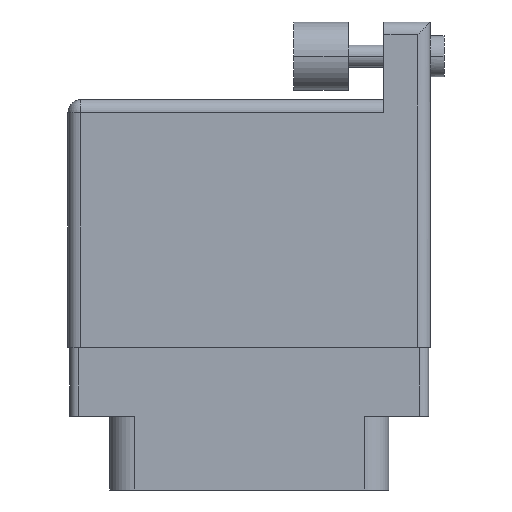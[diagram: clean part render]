
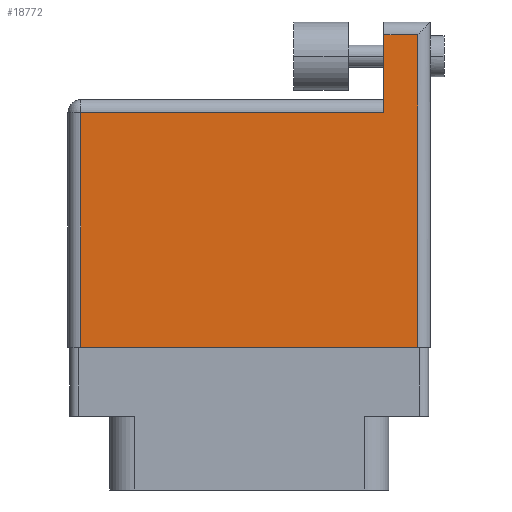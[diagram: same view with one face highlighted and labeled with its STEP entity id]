
A CAD part, front view. The second image highlights one B-rep face of the part: STEP entity #18772.
In plain terms, the highlighted face is planar.
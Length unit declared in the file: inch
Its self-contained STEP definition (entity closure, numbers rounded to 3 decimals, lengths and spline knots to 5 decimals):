
#295 = CARTESIAN_POINT ( 'NONE',  ( 0., 0.859, 0. ) ) ;
#579 = LINE ( 'NONE', #4725, #26224 ) ;
#1175 = CARTESIAN_POINT ( 'NONE',  ( 1.155, 0.859, 0. ) ) ;
#1245 = ORIENTED_EDGE ( 'NONE', *, *, #17087, .T. ) ;
#1353 = EDGE_LOOP ( 'NONE', ( #15851, #1245, #9022, #12493, #11175, #5600 ) ) ;
#1596 = LINE ( 'NONE', #13975, #12125 ) ;
#2258 = EDGE_CURVE ( 'NONE', #20447, #18096, #12729, .T. ) ;
#2852 = EDGE_CURVE ( 'NONE', #18024, #20447, #10308, .T. ) ;
#2933 = VECTOR ( 'NONE', #10618, 39.37008 ) ;
#4389 = EDGE_CURVE ( 'NONE', #18096, #18559, #22973, .T. ) ;
#4429 = DIRECTION ( 'NONE',  ( -1., 0., 0. ) ) ;
#4568 = VERTEX_POINT ( 'NONE', #19493 ) ;
#4725 = CARTESIAN_POINT ( 'NONE',  ( 1.155, 1.19, 0. ) ) ;
#5600 = ORIENTED_EDGE ( 'NONE', *, *, #2258, .T. ) ;
#5880 = VECTOR ( 'NONE', #19706, 39.37008 ) ;
#6705 = CARTESIAN_POINT ( 'NONE',  ( 1.278, 0., 0. ) ) ;
#6968 = DIRECTION ( 'NONE',  ( 0., 0., -1. ) ) ;
#7108 = PLANE ( 'NONE',  #9754 ) ;
#8918 = VECTOR ( 'NONE', #24708, 39.37008 ) ;
#9022 = ORIENTED_EDGE ( 'NONE', *, *, #14373, .T. ) ;
#9379 = CARTESIAN_POINT ( 'NONE',  ( 0., 0.906, 0. ) ) ;
#9754 = AXIS2_PLACEMENT_3D ( 'NONE', #9379, #6968, #15079 ) ;
#10308 = LINE ( 'NONE', #295, #16154 ) ;
#10618 = DIRECTION ( 'NONE',  ( 1., 0., 0. ) ) ;
#11175 = ORIENTED_EDGE ( 'NONE', *, *, #2852, .T. ) ;
#12125 = VECTOR ( 'NONE', #17682, 39.37008 ) ;
#12493 = ORIENTED_EDGE ( 'NONE', *, *, #24087, .T. ) ;
#12729 = LINE ( 'NONE', #20822, #8918 ) ;
#13600 = CARTESIAN_POINT ( 'NONE',  ( 1.278, 1.19, 0. ) ) ;
#13975 = CARTESIAN_POINT ( 'NONE',  ( 1.155, 1.143, 0. ) ) ;
#14122 = VERTEX_POINT ( 'NONE', #16762 ) ;
#14373 = EDGE_CURVE ( 'NONE', #4568, #14122, #1596, .T. ) ;
#15079 = DIRECTION ( 'NONE',  ( -1., 0., 0. ) ) ;
#15851 = ORIENTED_EDGE ( 'NONE', *, *, #4389, .T. ) ;
#16154 = VECTOR ( 'NONE', #4429, 39.37008 ) ;
#16762 = CARTESIAN_POINT ( 'NONE',  ( 1.155, 1.143, 0. ) ) ;
#16824 = DIRECTION ( 'NONE',  ( 0., -1., 0. ) ) ;
#17087 = EDGE_CURVE ( 'NONE', #18559, #4568, #17456, .T. ) ;
#17197 = CARTESIAN_POINT ( 'NONE',  ( 0.047, 0.859, 0. ) ) ;
#17456 = LINE ( 'NONE', #13600, #5880 ) ;
#17682 = DIRECTION ( 'NONE',  ( -1., 0., 0. ) ) ;
#18024 = VERTEX_POINT ( 'NONE', #1175 ) ;
#18096 = VERTEX_POINT ( 'NONE', #20165 ) ;
#18559 = VERTEX_POINT ( 'NONE', #6705 ) ;
#18772 = ADVANCED_FACE ( 'NONE', ( #25197 ), #7108, .F. ) ;
#19099 = CARTESIAN_POINT ( 'NONE',  ( 0., 0., 0. ) ) ;
#19493 = CARTESIAN_POINT ( 'NONE',  ( 1.278, 1.143, 0. ) ) ;
#19706 = DIRECTION ( 'NONE',  ( 0., 1., 0. ) ) ;
#20165 = CARTESIAN_POINT ( 'NONE',  ( 0.047, 0., 0. ) ) ;
#20447 = VERTEX_POINT ( 'NONE', #17197 ) ;
#20822 = CARTESIAN_POINT ( 'NONE',  ( 0.047, 0., 0. ) ) ;
#22973 = LINE ( 'NONE', #19099, #2933 ) ;
#24087 = EDGE_CURVE ( 'NONE', #14122, #18024, #579, .T. ) ;
#24708 = DIRECTION ( 'NONE',  ( 0., -1., 0. ) ) ;
#25197 = FACE_OUTER_BOUND ( 'NONE', #1353, .T. ) ;
#26224 = VECTOR ( 'NONE', #16824, 39.37008 ) ;
